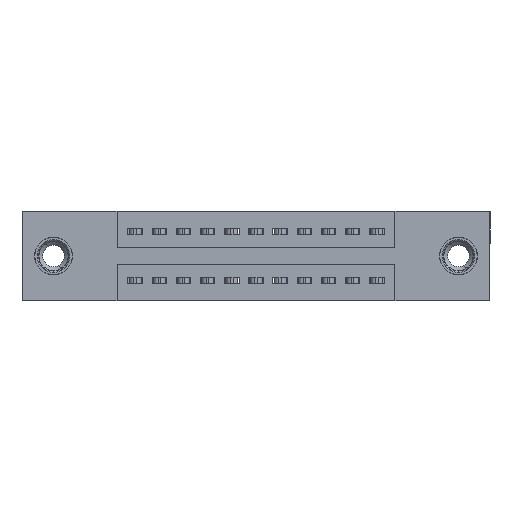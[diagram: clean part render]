
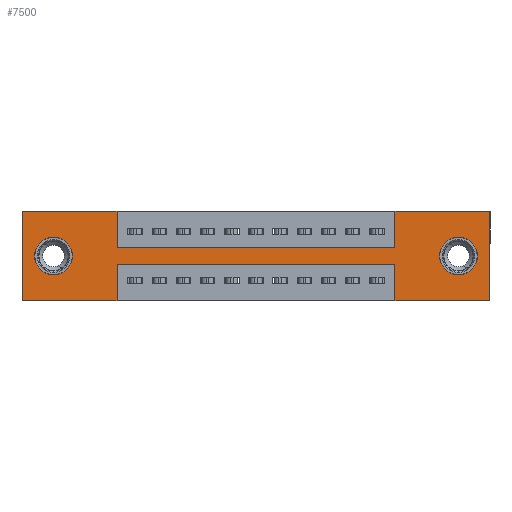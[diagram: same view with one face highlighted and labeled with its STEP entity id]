
A CAD part, front view. The second image highlights one B-rep face of the part: STEP entity #7500.
In plain terms, the highlighted planar face has unit normal (0, -1, 0).
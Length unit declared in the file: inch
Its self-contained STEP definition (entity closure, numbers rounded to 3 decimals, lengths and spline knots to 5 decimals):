
#2 = EDGE_CURVE ( 'NONE', #12902, #6581, #6310, .T. ) ;
#60 = EDGE_CURVE ( 'NONE', #1970, #9360, #17261, .T. ) ;
#86 = VECTOR ( 'NONE', #10645, 39.37008 ) ;
#132 = DIRECTION ( 'NONE',  ( 0., 0., -1. ) ) ;
#201 = PLANE ( 'NONE',  #2192 ) ;
#285 = ORIENTED_EDGE ( 'NONE', *, *, #14643, .F. ) ;
#310 = CARTESIAN_POINT ( 'NONE',  ( 0., 0., -0.37 ) ) ;
#452 = DIRECTION ( 'NONE',  ( 1., 0., 0. ) ) ;
#473 = VECTOR ( 'NONE', #863, 39.37008 ) ;
#479 = ORIENTED_EDGE ( 'NONE', *, *, #3282, .F. ) ;
#552 = EDGE_CURVE ( 'NONE', #9266, #9171, #5893, .T. ) ;
#617 = CARTESIAN_POINT ( 'NONE',  ( 1.805, 0., -0.263 ) ) ;
#656 = LINE ( 'NONE', #11202, #1083 ) ;
#812 = ORIENTED_EDGE ( 'NONE', *, *, #4225, .F. ) ;
#832 = EDGE_LOOP ( 'NONE', ( #14037, #8715 ) ) ;
#849 = VERTEX_POINT ( 'NONE', #11781 ) ;
#863 = DIRECTION ( 'NONE',  ( -1., 0., 0. ) ) ;
#941 = VERTEX_POINT ( 'NONE', #10372 ) ;
#967 = EDGE_CURVE ( 'NONE', #9003, #941, #8994, .T. ) ;
#1011 = DIRECTION ( 'NONE',  ( 0., 1., 0. ) ) ;
#1083 = VECTOR ( 'NONE', #7897, 39.37008 ) ;
#1252 = EDGE_CURVE ( 'NONE', #941, #9003, #1788, .T. ) ;
#1355 = LINE ( 'NONE', #13401, #86 ) ;
#1432 = CARTESIAN_POINT ( 'NONE',  ( 1.805, 0., -0.185 ) ) ;
#1440 = CARTESIAN_POINT ( 'NONE',  ( 0., 0., 0. ) ) ;
#1542 = ORIENTED_EDGE ( 'NONE', *, *, #4623, .T. ) ;
#1788 = CIRCLE ( 'NONE', #15046, 0.078 ) ;
#1928 = CARTESIAN_POINT ( 'NONE',  ( 1.805, 0., -0.185 ) ) ;
#1964 = CARTESIAN_POINT ( 'NONE',  ( 0.13, 0., -0.107 ) ) ;
#1970 = VERTEX_POINT ( 'NONE', #1440 ) ;
#2145 = LINE ( 'NONE', #14498, #473 ) ;
#2147 = CARTESIAN_POINT ( 'NONE',  ( 0.3925, 0., -0.37 ) ) ;
#2192 = AXIS2_PLACEMENT_3D ( 'NONE', #9613, #4233, #132 ) ;
#2296 = EDGE_CURVE ( 'NONE', #13007, #8192, #1355, .T. ) ;
#2462 = ORIENTED_EDGE ( 'NONE', *, *, #2296, .F. ) ;
#2633 = VECTOR ( 'NONE', #13108, 39.37008 ) ;
#3078 = CARTESIAN_POINT ( 'NONE',  ( 1.5425, 0., 0. ) ) ;
#3260 = LINE ( 'NONE', #5602, #14901 ) ;
#3282 = EDGE_CURVE ( 'NONE', #7350, #4345, #7651, .T. ) ;
#3425 = VERTEX_POINT ( 'NONE', #8830 ) ;
#3513 = EDGE_CURVE ( 'NONE', #8192, #5518, #2145, .T. ) ;
#3892 = EDGE_CURVE ( 'NONE', #6581, #3425, #11009, .T. ) ;
#4225 = EDGE_CURVE ( 'NONE', #4345, #9266, #656, .T. ) ;
#4233 = DIRECTION ( 'NONE',  ( 0., -1., 0. ) ) ;
#4345 = VERTEX_POINT ( 'NONE', #10727 ) ;
#4485 = VECTOR ( 'NONE', #9972, 39.37008 ) ;
#4525 = ORIENTED_EDGE ( 'NONE', *, *, #3513, .F. ) ;
#4623 = EDGE_CURVE ( 'NONE', #9301, #849, #14161, .T. ) ;
#4845 = DIRECTION ( 'NONE',  ( 0., 0., -1. ) ) ;
#5140 = VECTOR ( 'NONE', #9807, 39.37008 ) ;
#5518 = VERTEX_POINT ( 'NONE', #310 ) ;
#5587 = DIRECTION ( 'NONE',  ( 0., 1., 0. ) ) ;
#5602 = CARTESIAN_POINT ( 'NONE',  ( 0.3925, 0., -0.22 ) ) ;
#5627 = EDGE_CURVE ( 'NONE', #849, #9301, #10294, .T. ) ;
#5893 = LINE ( 'NONE', #7482, #9612 ) ;
#5913 = CARTESIAN_POINT ( 'NONE',  ( 0.3925, 0., 0. ) ) ;
#6058 = LINE ( 'NONE', #17075, #2633 ) ;
#6063 = AXIS2_PLACEMENT_3D ( 'NONE', #1432, #5587, #13710 ) ;
#6154 = FACE_OUTER_BOUND ( 'NONE', #7097, .T. ) ;
#6211 = DIRECTION ( 'NONE',  ( -1., 0., 0. ) ) ;
#6299 = CARTESIAN_POINT ( 'NONE',  ( 1.5425, 0., -0.22 ) ) ;
#6310 = LINE ( 'NONE', #10939, #7144 ) ;
#6355 = CARTESIAN_POINT ( 'NONE',  ( 0.3925, 0., -0.15 ) ) ;
#6498 = DIRECTION ( 'NONE',  ( 0., 1., 0. ) ) ;
#6581 = VERTEX_POINT ( 'NONE', #16712 ) ;
#6826 = ORIENTED_EDGE ( 'NONE', *, *, #2, .F. ) ;
#7097 = EDGE_LOOP ( 'NONE', ( #2462, #13954, #8970, #812, #479, #17513, #7393, #6826, #14723, #8726, #285, #4525 ) ) ;
#7144 = VECTOR ( 'NONE', #11057, 39.37008 ) ;
#7350 = VERTEX_POINT ( 'NONE', #9509 ) ;
#7393 = ORIENTED_EDGE ( 'NONE', *, *, #3892, .F. ) ;
#7482 = CARTESIAN_POINT ( 'NONE',  ( 1.5425, 0., -0.37 ) ) ;
#7500 = ADVANCED_FACE ( 'NONE', ( #15857, #16714, #6154 ), #201, .T. ) ;
#7651 = LINE ( 'NONE', #8515, #5140 ) ;
#7714 = CARTESIAN_POINT ( 'NONE',  ( 0.13, 0., -0.185 ) ) ;
#7744 = LINE ( 'NONE', #16694, #10042 ) ;
#7897 = DIRECTION ( 'NONE',  ( -1., 0., 0. ) ) ;
#8017 = DIRECTION ( 'NONE',  ( 1., 0., 0. ) ) ;
#8192 = VERTEX_POINT ( 'NONE', #2147 ) ;
#8286 = AXIS2_PLACEMENT_3D ( 'NONE', #1928, #12926, #4845 ) ;
#8515 = CARTESIAN_POINT ( 'NONE',  ( 1.935, 0., 0. ) ) ;
#8715 = ORIENTED_EDGE ( 'NONE', *, *, #1252, .T. ) ;
#8726 = ORIENTED_EDGE ( 'NONE', *, *, #60, .F. ) ;
#8830 = CARTESIAN_POINT ( 'NONE',  ( 1.5425, 0., 0. ) ) ;
#8874 = CARTESIAN_POINT ( 'NONE',  ( 0.3925, 0., -0.22 ) ) ;
#8970 = ORIENTED_EDGE ( 'NONE', *, *, #552, .F. ) ;
#8994 = CIRCLE ( 'NONE', #11973, 0.078 ) ;
#9003 = VERTEX_POINT ( 'NONE', #1964 ) ;
#9171 = VERTEX_POINT ( 'NONE', #6299 ) ;
#9266 = VERTEX_POINT ( 'NONE', #13328 ) ;
#9301 = VERTEX_POINT ( 'NONE', #617 ) ;
#9360 = VERTEX_POINT ( 'NONE', #5913 ) ;
#9509 = CARTESIAN_POINT ( 'NONE',  ( 1.935, 0., 0. ) ) ;
#9612 = VECTOR ( 'NONE', #12733, 39.37008 ) ;
#9613 = CARTESIAN_POINT ( 'NONE',  ( 0., 0., -0.37 ) ) ;
#9635 = VECTOR ( 'NONE', #452, 39.37008 ) ;
#9807 = DIRECTION ( 'NONE',  ( 0., 0., -1. ) ) ;
#9972 = DIRECTION ( 'NONE',  ( 0., 0., 1. ) ) ;
#10042 = VECTOR ( 'NONE', #11359, 39.37008 ) ;
#10294 = CIRCLE ( 'NONE', #6063, 0.078 ) ;
#10372 = CARTESIAN_POINT ( 'NONE',  ( 0.13, 0., -0.263 ) ) ;
#10410 = DIRECTION ( 'NONE',  ( 0., 0., 1. ) ) ;
#10645 = DIRECTION ( 'NONE',  ( 0., 0., -1. ) ) ;
#10727 = CARTESIAN_POINT ( 'NONE',  ( 1.935, 0., -0.37 ) ) ;
#10939 = CARTESIAN_POINT ( 'NONE',  ( 0.3925, 0., -0.15 ) ) ;
#11009 = LINE ( 'NONE', #3078, #4485 ) ;
#11057 = DIRECTION ( 'NONE',  ( 1., 0., 0. ) ) ;
#11202 = CARTESIAN_POINT ( 'NONE',  ( 0., 0., -0.37 ) ) ;
#11359 = DIRECTION ( 'NONE',  ( 0., 0., 1. ) ) ;
#11781 = CARTESIAN_POINT ( 'NONE',  ( 1.805, 0., -0.107 ) ) ;
#11899 = ORIENTED_EDGE ( 'NONE', *, *, #5627, .T. ) ;
#11973 = AXIS2_PLACEMENT_3D ( 'NONE', #7714, #1011, #10410 ) ;
#12134 = LINE ( 'NONE', #17483, #15128 ) ;
#12733 = DIRECTION ( 'NONE',  ( 0., 0., 1. ) ) ;
#12902 = VERTEX_POINT ( 'NONE', #6355 ) ;
#12926 = DIRECTION ( 'NONE',  ( 0., 1., 0. ) ) ;
#13007 = VERTEX_POINT ( 'NONE', #8874 ) ;
#13108 = DIRECTION ( 'NONE',  ( 0., 0., -1. ) ) ;
#13328 = CARTESIAN_POINT ( 'NONE',  ( 1.5425, 0., -0.37 ) ) ;
#13401 = CARTESIAN_POINT ( 'NONE',  ( 0.3925, 0., -0.37 ) ) ;
#13710 = DIRECTION ( 'NONE',  ( 0., 0., -1. ) ) ;
#13954 = ORIENTED_EDGE ( 'NONE', *, *, #15839, .F. ) ;
#14037 = ORIENTED_EDGE ( 'NONE', *, *, #967, .T. ) ;
#14161 = CIRCLE ( 'NONE', #8286, 0.078 ) ;
#14498 = CARTESIAN_POINT ( 'NONE',  ( 0., 0., -0.37 ) ) ;
#14561 = CARTESIAN_POINT ( 'NONE',  ( 0.13, 0., -0.185 ) ) ;
#14643 = EDGE_CURVE ( 'NONE', #5518, #1970, #7744, .T. ) ;
#14708 = CARTESIAN_POINT ( 'NONE',  ( 0., 0., 0. ) ) ;
#14723 = ORIENTED_EDGE ( 'NONE', *, *, #15505, .F. ) ;
#14901 = VECTOR ( 'NONE', #6211, 39.37008 ) ;
#15046 = AXIS2_PLACEMENT_3D ( 'NONE', #14561, #6498, #17282 ) ;
#15128 = VECTOR ( 'NONE', #8017, 39.37008 ) ;
#15505 = EDGE_CURVE ( 'NONE', #9360, #12902, #6058, .T. ) ;
#15665 = EDGE_CURVE ( 'NONE', #3425, #7350, #12134, .T. ) ;
#15839 = EDGE_CURVE ( 'NONE', #9171, #13007, #3260, .T. ) ;
#15857 = FACE_BOUND ( 'NONE', #17223, .T. ) ;
#16694 = CARTESIAN_POINT ( 'NONE',  ( 0., 0., 0. ) ) ;
#16712 = CARTESIAN_POINT ( 'NONE',  ( 1.5425, 0., -0.15 ) ) ;
#16714 = FACE_BOUND ( 'NONE', #832, .T. ) ;
#17075 = CARTESIAN_POINT ( 'NONE',  ( 0.3925, 0., 0. ) ) ;
#17223 = EDGE_LOOP ( 'NONE', ( #11899, #1542 ) ) ;
#17261 = LINE ( 'NONE', #14708, #9635 ) ;
#17282 = DIRECTION ( 'NONE',  ( 0., 0., 1. ) ) ;
#17483 = CARTESIAN_POINT ( 'NONE',  ( 0., 0., 0. ) ) ;
#17513 = ORIENTED_EDGE ( 'NONE', *, *, #15665, .F. ) ;
